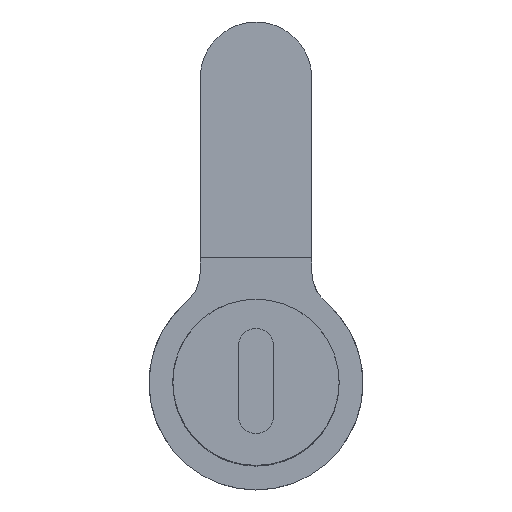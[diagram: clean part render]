
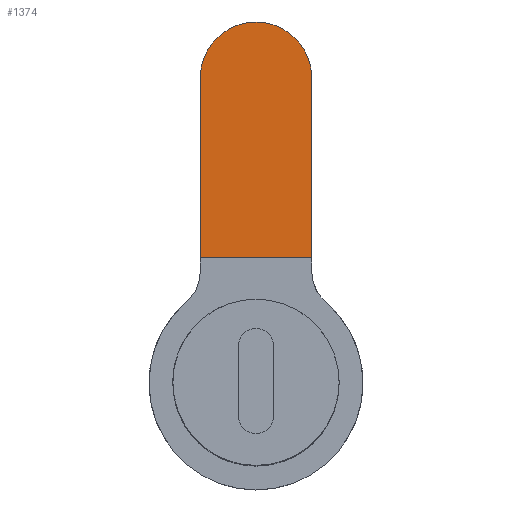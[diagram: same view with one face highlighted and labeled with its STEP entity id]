
A CAD part, top view. The second image highlights one B-rep face of the part: STEP entity #1374.
In plain terms, the highlighted planar face has unit normal (0, 0, 1).
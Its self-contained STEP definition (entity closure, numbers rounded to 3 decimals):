
#190=LINE('',#2973,#263);
#199=LINE('',#2990,#272);
#201=LINE('',#3002,#274);
#263=VECTOR('',#1870,10.262);
#272=VECTOR('',#1885,10.262);
#274=VECTOR('',#1907,6.35);
#303=PLANE('',#1538);
#383=FACE_OUTER_BOUND('',#469,.T.);
#469=EDGE_LOOP('',(#1290,#1291,#1292,#1293));
#540=CIRCLE('',#1526,3.175);
#672=VERTEX_POINT('',#2970);
#673=VERTEX_POINT('',#2972);
#676=VERTEX_POINT('',#2981);
#678=VERTEX_POINT('',#2988);
#868=EDGE_CURVE('',#672,#673,#190,.T.);
#874=EDGE_CURVE('',#676,#672,#540,.T.);
#878=EDGE_CURVE('',#676,#678,#199,.T.);
#883=EDGE_CURVE('',#678,#673,#201,.T.);
#1290=ORIENTED_EDGE('',*,*,#883,.T.);
#1291=ORIENTED_EDGE('',*,*,#868,.F.);
#1292=ORIENTED_EDGE('',*,*,#874,.F.);
#1293=ORIENTED_EDGE('',*,*,#878,.T.);
#1374=ADVANCED_FACE('',(#383),#303,.T.);
#1526=AXIS2_PLACEMENT_3D('',#2983,#1878,#1879);
#1538=AXIS2_PLACEMENT_3D('',#3003,#1908,#1909);
#1870=DIRECTION('',(0.,-1.,0.));
#1878=DIRECTION('center_axis',(0.,0.,
-1.));
#1879=DIRECTION('ref_axis',(-1.,0.,0.));
#1885=DIRECTION('',(0.,-1.,0.));
#1907=DIRECTION('',(1.,0.,0.));
#1908=DIRECTION('center_axis',(0.,0.,
1.));
#1909=DIRECTION('ref_axis',(0.,-1.,0.));
#2970=CARTESIAN_POINT('',(-11.75,17.399,16.698));
#2972=CARTESIAN_POINT('',(-11.75,7.137,16.698));
#2973=CARTESIAN_POINT('',(-11.75,17.399,16.698));
#2981=CARTESIAN_POINT('',(-18.1,17.399,16.698));
#2983=CARTESIAN_POINT('Origin',(-14.925,17.399,16.698));
#2988=CARTESIAN_POINT('',(-18.1,7.137,16.698));
#2990=CARTESIAN_POINT('',(-18.1,17.399,16.698));
#3002=CARTESIAN_POINT('',(-18.1,7.137,16.698));
#3003=CARTESIAN_POINT('Origin',(-14.925,0.,
16.698));
